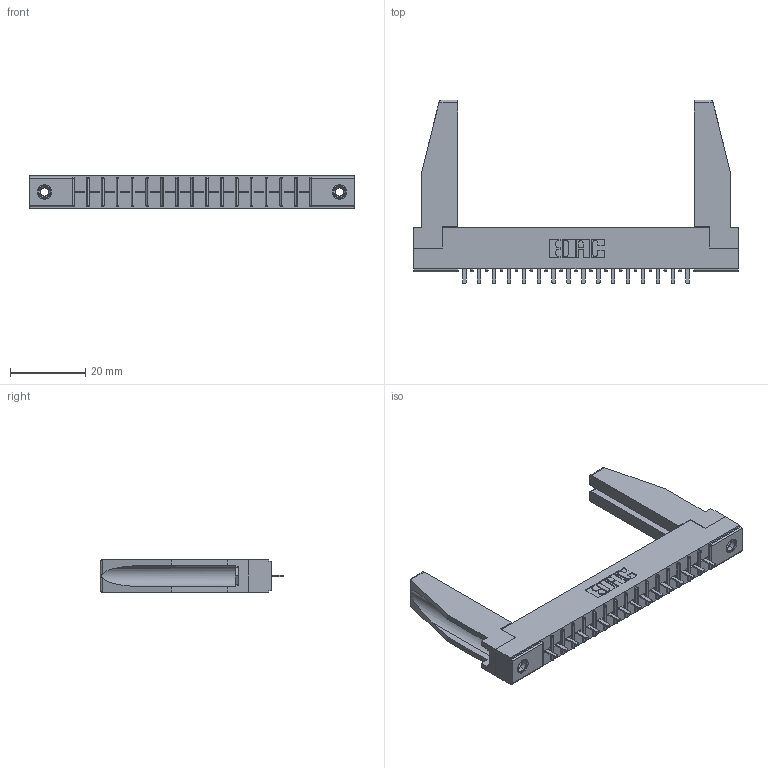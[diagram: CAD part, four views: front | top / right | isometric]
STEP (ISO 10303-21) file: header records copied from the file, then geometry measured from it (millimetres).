
FILE_DESCRIPTION (( 'STEP AP203' ), '1' );
FILE_NAME ('316-016-521-178.STEP', '2018-07-31T01:03:19', ( '' ), ( '' ), 'SwSTEP 2.0', 'SolidWorks 2016', '' );
FILE_SCHEMA (( 'CONFIG_CONTROL_DESIGN' ));
Length unit declared in the file: inch
Products named in the file (5): 306 Part_.156 Dia; 306-290-001_121; 345-250-001_345-250-001-102; 307-220-078; 316-016-521-178
Assembly tree (21 placements, depth 2):
  316-016-521-178
    306 Part_.156 Dia
    306-290-001_121  x16
    345-250-001_345-250-001-102  x2
    307-220-078  x2
Bounding box: 86.41 x 48.92 x 8.71 mm (x, y, z)
Volume: 9860.1 mm3; surface area: 12193.5 mm2
Topology: 21 solids, 21 shells, 1366 faces, 3798 edges, 2436 vertices
Faces by surface type: plane 904, cylinder 382, sphere 64, cone 12, torus 4
Entity records: 20684 total; most frequent: CARTESIAN_POINT 3469, ORIENTED_EDGE 3394, DIRECTION 3375, EDGE_CURVE 1697, VECTOR 1315, LINE 1315, VERTEX_POINT 1082, AXIS2_PLACEMENT_3D 1030
